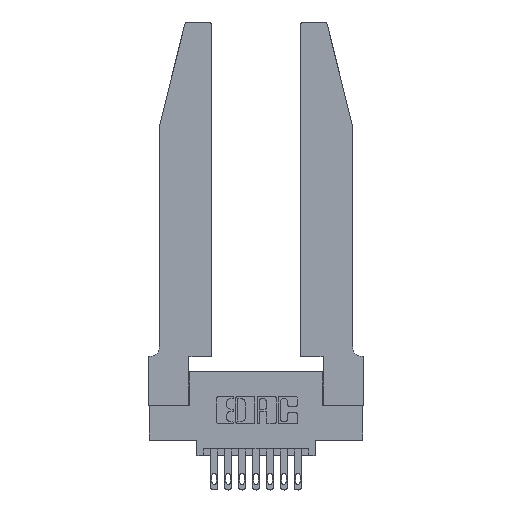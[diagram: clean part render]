
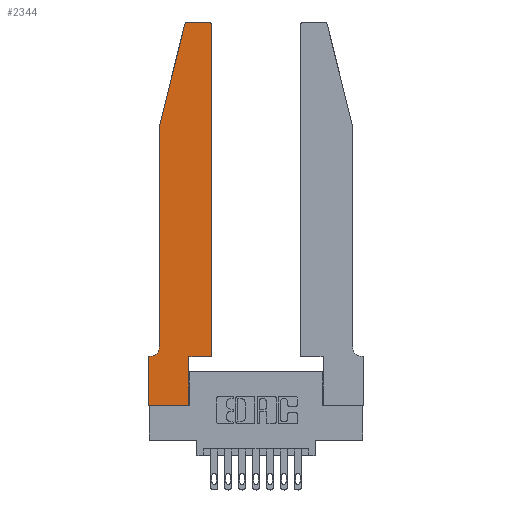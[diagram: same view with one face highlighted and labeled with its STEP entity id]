
A CAD part, top view. The second image highlights one B-rep face of the part: STEP entity #2344.
In plain terms, the highlighted planar face has unit normal (0, 0, 1).
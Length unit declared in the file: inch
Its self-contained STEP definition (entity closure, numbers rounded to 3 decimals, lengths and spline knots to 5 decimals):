
#85 = EDGE_CURVE ( 'NONE', #8300, #10365, #12653, .T. ) ;
#132 = EDGE_CURVE ( 'NONE', #12710, #9342, #9184, .T. ) ;
#199 = DIRECTION ( 'NONE',  ( 0., 1., 0. ) ) ;
#203 = CARTESIAN_POINT ( 'NONE',  ( 0.2865, 0., 0.37 ) ) ;
#238 = VERTEX_POINT ( 'NONE', #3283 ) ;
#351 = ORIENTED_EDGE ( 'NONE', *, *, #12956, .T. ) ;
#465 = CIRCLE ( 'NONE', #14823, 0.03 ) ;
#568 = LINE ( 'NONE', #4958, #12031 ) ;
#592 = AXIS2_PLACEMENT_3D ( 'NONE', #12662, #1056, #3516 ) ;
#985 = CARTESIAN_POINT ( 'NONE',  ( 0.4505, 0.35, 0.37 ) ) ;
#997 = ORIENTED_EDGE ( 'NONE', *, *, #9563, .T. ) ;
#1056 = DIRECTION ( 'NONE',  ( 0., 0., 1. ) ) ;
#1089 = DIRECTION ( 'NONE',  ( 0., -1., 0. ) ) ;
#1096 = DIRECTION ( 'NONE',  ( 0., 0., 1. ) ) ;
#1328 = VERTEX_POINT ( 'NONE', #9242 ) ;
#1462 = CIRCLE ( 'NONE', #3628, 0.03 ) ;
#1677 = LINE ( 'NONE', #8753, #2227 ) ;
#1692 = VERTEX_POINT ( 'NONE', #4085 ) ;
#2051 = EDGE_CURVE ( 'NONE', #238, #6307, #568, .T. ) ;
#2227 = VECTOR ( 'NONE', #5419, 39.37008 ) ;
#2285 = LINE ( 'NONE', #8079, #13904 ) ;
#2302 = DIRECTION ( 'NONE',  ( 1., 0., 0. ) ) ;
#2344 = ADVANCED_FACE ( 'NONE', ( #5836 ), #11489, .T. ) ;
#2473 = LINE ( 'NONE', #8415, #5001 ) ;
#2723 = VERTEX_POINT ( 'NONE', #3553 ) ;
#2728 = AXIS2_PLACEMENT_3D ( 'NONE', #3077, #7649, #7754 ) ;
#2734 = CARTESIAN_POINT ( 'NONE',  ( 0.0055, 0.35, 0.37 ) ) ;
#3065 = ORIENTED_EDGE ( 'NONE', *, *, #85, .T. ) ;
#3077 = CARTESIAN_POINT ( 'NONE',  ( 0.0055, 0.42, 0.37 ) ) ;
#3274 = CARTESIAN_POINT ( 'NONE',  ( 0.0755, 2., 0.37 ) ) ;
#3283 = CARTESIAN_POINT ( 'NONE',  ( 0., 0.35, 0.37 ) ) ;
#3302 = VECTOR ( 'NONE', #3984, 39.37008 ) ;
#3516 = DIRECTION ( 'NONE',  ( 1., 0., 0. ) ) ;
#3553 = CARTESIAN_POINT ( 'NONE',  ( 0.25487, 2.72718, 0.37 ) ) ;
#3628 = AXIS2_PLACEMENT_3D ( 'NONE', #9283, #15026, #2302 ) ;
#3980 = ORIENTED_EDGE ( 'NONE', *, *, #14859, .T. ) ;
#3984 = DIRECTION ( 'NONE',  ( -1., 0., 0. ) ) ;
#4085 = CARTESIAN_POINT ( 'NONE',  ( 0.4205, 2.75, 0.37 ) ) ;
#4160 = VERTEX_POINT ( 'NONE', #13234 ) ;
#4958 = CARTESIAN_POINT ( 'NONE',  ( 0., 0., 0.37 ) ) ;
#5001 = VECTOR ( 'NONE', #199, 39.37008 ) ;
#5419 = DIRECTION ( 'NONE',  ( -1., 0., 0. ) ) ;
#5601 = EDGE_CURVE ( 'NONE', #13256, #1328, #2473, .T. ) ;
#5776 = ORIENTED_EDGE ( 'NONE', *, *, #2051, .T. ) ;
#5814 = CARTESIAN_POINT ( 'NONE',  ( 0.284, 2.72, 0.37 ) ) ;
#5836 = FACE_OUTER_BOUND ( 'NONE', #11966, .T. ) ;
#5986 = EDGE_CURVE ( 'NONE', #4160, #2723, #465, .T. ) ;
#6194 = VECTOR ( 'NONE', #10254, 39.37008 ) ;
#6307 = VERTEX_POINT ( 'NONE', #11653 ) ;
#6423 = EDGE_CURVE ( 'NONE', #9132, #12710, #2285, .T. ) ;
#6636 = CARTESIAN_POINT ( 'NONE',  ( 0.2865, 0.35, 0.37 ) ) ;
#6657 = ORIENTED_EDGE ( 'NONE', *, *, #10804, .T. ) ;
#7188 = VECTOR ( 'NONE', #8985, 39.37008 ) ;
#7524 = ORIENTED_EDGE ( 'NONE', *, *, #132, .T. ) ;
#7649 = DIRECTION ( 'NONE',  ( 0., 0., -1. ) ) ;
#7754 = DIRECTION ( 'NONE',  ( -1., 0., 0. ) ) ;
#8079 = CARTESIAN_POINT ( 'NONE',  ( 0.0755, 2., 0.37 ) ) ;
#8295 = DIRECTION ( 'NONE',  ( 0., -1., 0. ) ) ;
#8300 = VERTEX_POINT ( 'NONE', #203 ) ;
#8415 = CARTESIAN_POINT ( 'NONE',  ( 0.4505, 0.35, 0.37 ) ) ;
#8509 = ORIENTED_EDGE ( 'NONE', *, *, #5986, .T. ) ;
#8589 = CARTESIAN_POINT ( 'NONE',  ( 0.0755, 2., 0.37 ) ) ;
#8753 = CARTESIAN_POINT ( 'NONE',  ( 0.0755, 0.35, 0.37 ) ) ;
#8985 = DIRECTION ( 'NONE',  ( 0., 1., 0. ) ) ;
#9128 = DIRECTION ( 'NONE',  ( 1., 0., 0. ) ) ;
#9132 = VERTEX_POINT ( 'NONE', #8589 ) ;
#9134 = EDGE_CURVE ( 'NONE', #10365, #13256, #13474, .T. ) ;
#9184 = CIRCLE ( 'NONE', #2728, 0.07 ) ;
#9242 = CARTESIAN_POINT ( 'NONE',  ( 0.4505, 2.72, 0.37 ) ) ;
#9243 = DIRECTION ( 'NONE',  ( 1., 0., 0. ) ) ;
#9283 = CARTESIAN_POINT ( 'NONE',  ( 0.4205, 2.72, 0.37 ) ) ;
#9342 = VERTEX_POINT ( 'NONE', #2734 ) ;
#9563 = EDGE_CURVE ( 'NONE', #1692, #4160, #11117, .T. ) ;
#9646 = CARTESIAN_POINT ( 'NONE',  ( 0.0755, 0.42, 0.37 ) ) ;
#10254 = DIRECTION ( 'NONE',  ( 1., 0., 0. ) ) ;
#10365 = VERTEX_POINT ( 'NONE', #11288 ) ;
#10730 = CARTESIAN_POINT ( 'NONE',  ( 0.4505, 0.35, 0.37 ) ) ;
#10804 = EDGE_CURVE ( 'NONE', #9342, #238, #1677, .T. ) ;
#11117 = LINE ( 'NONE', #13278, #3302 ) ;
#11288 = CARTESIAN_POINT ( 'NONE',  ( 0.2865, 0.35, 0.37 ) ) ;
#11478 = ORIENTED_EDGE ( 'NONE', *, *, #11663, .T. ) ;
#11489 = PLANE ( 'NONE',  #592 ) ;
#11507 = CARTESIAN_POINT ( 'NONE',  ( 0., 0., 0.37 ) ) ;
#11653 = CARTESIAN_POINT ( 'NONE',  ( 0., 0., 0.37 ) ) ;
#11663 = EDGE_CURVE ( 'NONE', #1328, #1692, #1462, .T. ) ;
#11966 = EDGE_LOOP ( 'NONE', ( #997, #8509, #351, #12696, #7524, #6657, #5776, #3980, #3065, #12717, #13705, #11478 ) ) ;
#12031 = VECTOR ( 'NONE', #8295, 39.37008 ) ;
#12075 = VECTOR ( 'NONE', #12574, 39.37008 ) ;
#12297 = VECTOR ( 'NONE', #9128, 39.37008 ) ;
#12574 = DIRECTION ( 'NONE',  ( -0.239, -0.971, 0. ) ) ;
#12653 = LINE ( 'NONE', #6636, #7188 ) ;
#12662 = CARTESIAN_POINT ( 'NONE',  ( 0., 0.35, 0.37 ) ) ;
#12696 = ORIENTED_EDGE ( 'NONE', *, *, #6423, .T. ) ;
#12710 = VERTEX_POINT ( 'NONE', #9646 ) ;
#12717 = ORIENTED_EDGE ( 'NONE', *, *, #9134, .T. ) ;
#12733 = LINE ( 'NONE', #3274, #12075 ) ;
#12956 = EDGE_CURVE ( 'NONE', #2723, #9132, #12733, .T. ) ;
#13234 = CARTESIAN_POINT ( 'NONE',  ( 0.284, 2.75, 0.37 ) ) ;
#13256 = VERTEX_POINT ( 'NONE', #10730 ) ;
#13278 = CARTESIAN_POINT ( 'NONE',  ( 0.2605, 2.75, 0.37 ) ) ;
#13474 = LINE ( 'NONE', #985, #6194 ) ;
#13705 = ORIENTED_EDGE ( 'NONE', *, *, #5601, .T. ) ;
#13904 = VECTOR ( 'NONE', #1089, 39.37008 ) ;
#14628 = LINE ( 'NONE', #11507, #12297 ) ;
#14823 = AXIS2_PLACEMENT_3D ( 'NONE', #5814, #1096, #9243 ) ;
#14859 = EDGE_CURVE ( 'NONE', #6307, #8300, #14628, .T. ) ;
#15026 = DIRECTION ( 'NONE',  ( 0., 0., 1. ) ) ;
